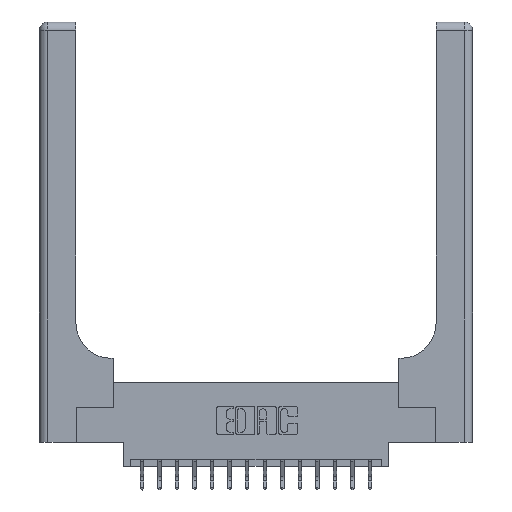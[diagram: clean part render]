
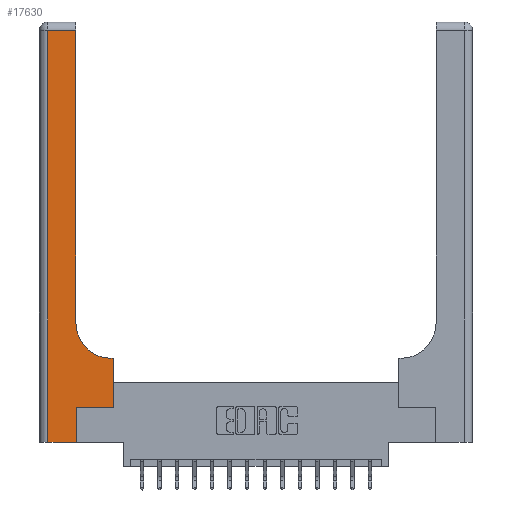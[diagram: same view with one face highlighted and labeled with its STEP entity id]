
A CAD part, top view. The second image highlights one B-rep face of the part: STEP entity #17630.
In plain terms, the highlighted planar face has unit normal (0, 0, 1).
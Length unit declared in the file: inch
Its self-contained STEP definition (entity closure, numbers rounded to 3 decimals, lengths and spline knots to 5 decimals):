
#466 = DIRECTION ( 'NONE',  ( 0., -1., 0. ) ) ;
#563 = EDGE_CURVE ( 'NONE', #6798, #13788, #17305, .T. ) ;
#764 = CARTESIAN_POINT ( 'NONE',  ( 0., 0., 0.37 ) ) ;
#966 = CIRCLE ( 'NONE', #6850, 0.25 ) ;
#1145 = DIRECTION ( 'NONE',  ( 1., 0., 0. ) ) ;
#2083 = CARTESIAN_POINT ( 'NONE',  ( 0.26, 0.6, 0.37 ) ) ;
#2113 = VERTEX_POINT ( 'NONE', #16873 ) ;
#2216 = DIRECTION ( 'NONE',  ( 1., 0., 0. ) ) ;
#2312 = EDGE_CURVE ( 'NONE', #2113, #7794, #3212, .T. ) ;
#2695 = EDGE_CURVE ( 'NONE', #14543, #11824, #966, .T. ) ;
#2765 = VERTEX_POINT ( 'NONE', #5840 ) ;
#3112 = VECTOR ( 'NONE', #1145, 39.37008 ) ;
#3212 = LINE ( 'NONE', #17480, #13955 ) ;
#3213 = DIRECTION ( 'NONE',  ( -1., 0., 0. ) ) ;
#3490 = CARTESIAN_POINT ( 'NONE',  ( 0.265, 0., 0.37 ) ) ;
#3558 = LINE ( 'NONE', #5517, #3112 ) ;
#3575 = LINE ( 'NONE', #13919, #10749 ) ;
#3600 = EDGE_CURVE ( 'NONE', #9408, #14543, #13267, .T. ) ;
#4115 = ORIENTED_EDGE ( 'NONE', *, *, #10129, .T. ) ;
#4261 = ORIENTED_EDGE ( 'NONE', *, *, #9304, .T. ) ;
#4270 = CARTESIAN_POINT ( 'NONE',  ( 0.51, 0.85, 0.37 ) ) ;
#4285 = VECTOR ( 'NONE', #17508, 39.37008 ) ;
#4828 = CARTESIAN_POINT ( 'NONE',  ( 0.26, 0.85, 0.37 ) ) ;
#4994 = DIRECTION ( 'NONE',  ( -1., 0., 0. ) ) ;
#5517 = CARTESIAN_POINT ( 'NONE',  ( 0.265, 0.25, 0.37 ) ) ;
#5672 = EDGE_CURVE ( 'NONE', #11824, #2113, #15627, .T. ) ;
#5700 = VECTOR ( 'NONE', #4994, 39.37008 ) ;
#5727 = DIRECTION ( 'NONE',  ( 1., 0., 0. ) ) ;
#5840 = CARTESIAN_POINT ( 'NONE',  ( 0.528, 0.25, 0.37 ) ) ;
#5920 = ORIENTED_EDGE ( 'NONE', *, *, #9628, .T. ) ;
#5983 = VECTOR ( 'NONE', #2216, 39.37008 ) ;
#6024 = ORIENTED_EDGE ( 'NONE', *, *, #2312, .T. ) ;
#6049 = CARTESIAN_POINT ( 'NONE',  ( 0., 3., 0.37 ) ) ;
#6793 = VECTOR ( 'NONE', #466, 39.37008 ) ;
#6798 = VERTEX_POINT ( 'NONE', #14064 ) ;
#6850 = AXIS2_PLACEMENT_3D ( 'NONE', #4270, #14233, #5727 ) ;
#7641 = CARTESIAN_POINT ( 'NONE',  ( 0.06, 3., 0.37 ) ) ;
#7696 = LINE ( 'NONE', #7641, #6793 ) ;
#7794 = VERTEX_POINT ( 'NONE', #10750 ) ;
#7986 = EDGE_LOOP ( 'NONE', ( #10920, #6024, #14206, #14744, #4261, #4115, #5920, #15454, #9532 ) ) ;
#8099 = LINE ( 'NONE', #9028, #4285 ) ;
#9028 = CARTESIAN_POINT ( 'NONE',  ( 0.265, 0., 0.37 ) ) ;
#9304 = EDGE_CURVE ( 'NONE', #13788, #14382, #8099, .T. ) ;
#9408 = VERTEX_POINT ( 'NONE', #14854 ) ;
#9532 = ORIENTED_EDGE ( 'NONE', *, *, #2695, .T. ) ;
#9628 = EDGE_CURVE ( 'NONE', #2765, #9408, #3575, .T. ) ;
#9761 = DIRECTION ( 'NONE',  ( 0., 1., 0. ) ) ;
#9945 = CARTESIAN_POINT ( 'NONE',  ( 0.26, 3., 0.37 ) ) ;
#10129 = EDGE_CURVE ( 'NONE', #14382, #2765, #3558, .T. ) ;
#10363 = PLANE ( 'NONE',  #16072 ) ;
#10749 = VECTOR ( 'NONE', #9761, 39.37008 ) ;
#10750 = CARTESIAN_POINT ( 'NONE',  ( 0.06, 2.94, 0.37 ) ) ;
#10920 = ORIENTED_EDGE ( 'NONE', *, *, #5672, .T. ) ;
#11780 = DIRECTION ( 'NONE',  ( 0., 0., -1. ) ) ;
#11824 = VERTEX_POINT ( 'NONE', #4828 ) ;
#12291 = VECTOR ( 'NONE', #12828, 39.37008 ) ;
#12828 = DIRECTION ( 'NONE',  ( 0., 1., 0. ) ) ;
#13179 = DIRECTION ( 'NONE',  ( -1., 0., 0. ) ) ;
#13267 = LINE ( 'NONE', #2083, #5700 ) ;
#13700 = EDGE_CURVE ( 'NONE', #7794, #6798, #7696, .T. ) ;
#13788 = VERTEX_POINT ( 'NONE', #3490 ) ;
#13919 = CARTESIAN_POINT ( 'NONE',  ( 0.528, 0.25, 0.37 ) ) ;
#13955 = VECTOR ( 'NONE', #13179, 39.37008 ) ;
#14064 = CARTESIAN_POINT ( 'NONE',  ( 0.06, 0., 0.37 ) ) ;
#14206 = ORIENTED_EDGE ( 'NONE', *, *, #13700, .T. ) ;
#14233 = DIRECTION ( 'NONE',  ( 0., 0., -1. ) ) ;
#14382 = VERTEX_POINT ( 'NONE', #17777 ) ;
#14543 = VERTEX_POINT ( 'NONE', #15307 ) ;
#14744 = ORIENTED_EDGE ( 'NONE', *, *, #563, .T. ) ;
#14854 = CARTESIAN_POINT ( 'NONE',  ( 0.528, 0.6, 0.37 ) ) ;
#15307 = CARTESIAN_POINT ( 'NONE',  ( 0.51, 0.6, 0.37 ) ) ;
#15454 = ORIENTED_EDGE ( 'NONE', *, *, #3600, .T. ) ;
#15627 = LINE ( 'NONE', #9945, #12291 ) ;
#16072 = AXIS2_PLACEMENT_3D ( 'NONE', #6049, #11780, #3213 ) ;
#16873 = CARTESIAN_POINT ( 'NONE',  ( 0.26, 2.94, 0.37 ) ) ;
#17305 = LINE ( 'NONE', #764, #5983 ) ;
#17480 = CARTESIAN_POINT ( 'NONE',  ( 0., 2.94, 0.37 ) ) ;
#17508 = DIRECTION ( 'NONE',  ( 0., 1., 0. ) ) ;
#17630 = ADVANCED_FACE ( 'NONE', ( #17751 ), #10363, .F. ) ;
#17751 = FACE_OUTER_BOUND ( 'NONE', #7986, .T. ) ;
#17777 = CARTESIAN_POINT ( 'NONE',  ( 0.265, 0.25, 0.37 ) ) ;
